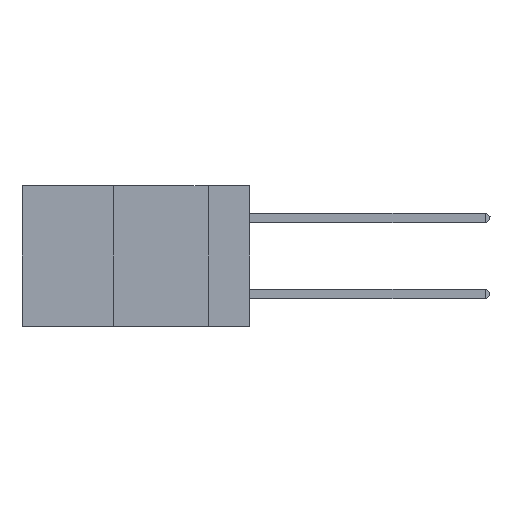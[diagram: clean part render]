
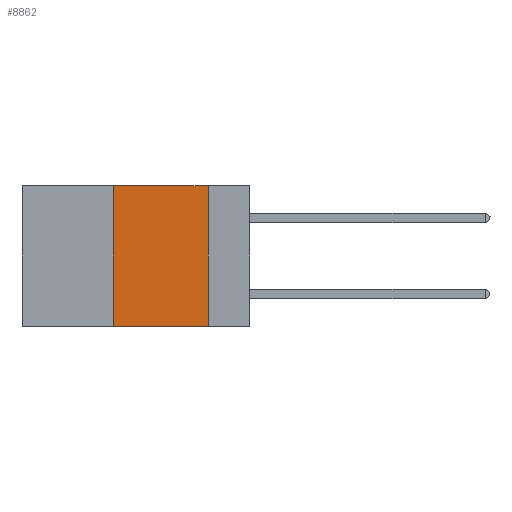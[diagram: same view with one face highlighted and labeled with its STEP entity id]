
A CAD part, left-side view. The second image highlights one B-rep face of the part: STEP entity #8862.
In plain terms, the highlighted planar face has unit normal (-1, 0, 0).
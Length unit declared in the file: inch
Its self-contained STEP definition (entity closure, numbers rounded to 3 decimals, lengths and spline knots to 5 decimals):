
#1822 = CARTESIAN_POINT ( 'NONE',  ( 0., 0.6, 0. ) ) ;
#1891 = EDGE_CURVE ( 'NONE', #4380, #4237, #18256, .T. ) ;
#3250 = ORIENTED_EDGE ( 'NONE', *, *, #12107, .T. ) ;
#3522 = VECTOR ( 'NONE', #9834, 39.37008 ) ;
#3561 = ORIENTED_EDGE ( 'NONE', *, *, #4230, .F. ) ;
#4230 = EDGE_CURVE ( 'NONE', #4237, #5677, #7608, .T. ) ;
#4237 = VERTEX_POINT ( 'NONE', #23784 ) ;
#4380 = VERTEX_POINT ( 'NONE', #20194 ) ;
#5677 = VERTEX_POINT ( 'NONE', #25842 ) ;
#6286 = DIRECTION ( 'NONE',  ( 1., 0., 0. ) ) ;
#6962 = VECTOR ( 'NONE', #11979, 39.37008 ) ;
#7425 = DIRECTION ( 'NONE',  ( 0., 0., -1. ) ) ;
#7608 = LINE ( 'NONE', #1822, #6962 ) ;
#8862 = ADVANCED_FACE ( 'NONE', ( #12331 ), #21995, .F. ) ;
#9146 = CARTESIAN_POINT ( 'NONE',  ( 0., 0.11, -0.37 ) ) ;
#9359 = DIRECTION ( 'NONE',  ( 0., -1., 0. ) ) ;
#9783 = LINE ( 'NONE', #17296, #22335 ) ;
#9834 = DIRECTION ( 'NONE',  ( 0., 0., 1. ) ) ;
#10286 = CARTESIAN_POINT ( 'NONE',  ( 0., 0.6, 0. ) ) ;
#11471 = EDGE_CURVE ( 'NONE', #5677, #23271, #9783, .T. ) ;
#11979 = DIRECTION ( 'NONE',  ( 0., -1., 0. ) ) ;
#12107 = EDGE_CURVE ( 'NONE', #4380, #23271, #22602, .T. ) ;
#12149 = ORIENTED_EDGE ( 'NONE', *, *, #1891, .F. ) ;
#12331 = FACE_OUTER_BOUND ( 'NONE', #24675, .T. ) ;
#13654 = AXIS2_PLACEMENT_3D ( 'NONE', #10286, #6286, #20124 ) ;
#17176 = CARTESIAN_POINT ( 'NONE',  ( 0., 0.6, -0.37 ) ) ;
#17296 = CARTESIAN_POINT ( 'NONE',  ( 0., 0.11, 0. ) ) ;
#17420 = VECTOR ( 'NONE', #9359, 39.37008 ) ;
#18256 = LINE ( 'NONE', #21563, #3522 ) ;
#18289 = ORIENTED_EDGE ( 'NONE', *, *, #11471, .F. ) ;
#20124 = DIRECTION ( 'NONE',  ( 0., 0., -1. ) ) ;
#20194 = CARTESIAN_POINT ( 'NONE',  ( 0., 0.36, -0.37 ) ) ;
#21563 = CARTESIAN_POINT ( 'NONE',  ( 0., 0.36, 0. ) ) ;
#21995 = PLANE ( 'NONE',  #13654 ) ;
#22335 = VECTOR ( 'NONE', #7425, 39.37008 ) ;
#22602 = LINE ( 'NONE', #17176, #17420 ) ;
#23271 = VERTEX_POINT ( 'NONE', #9146 ) ;
#23784 = CARTESIAN_POINT ( 'NONE',  ( 0., 0.36, 0. ) ) ;
#24675 = EDGE_LOOP ( 'NONE', ( #18289, #3561, #12149, #3250 ) ) ;
#25842 = CARTESIAN_POINT ( 'NONE',  ( 0., 0.11, 0. ) ) ;
